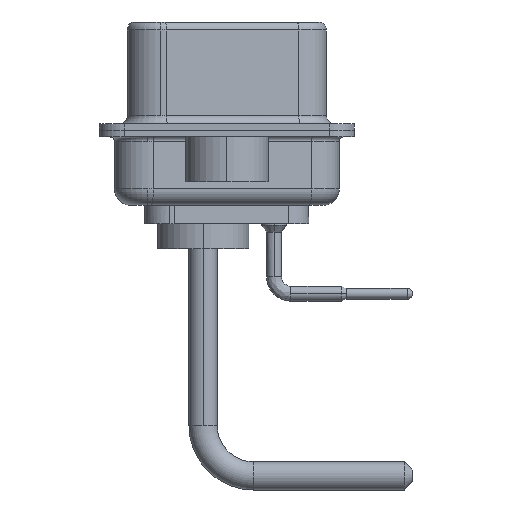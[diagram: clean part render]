
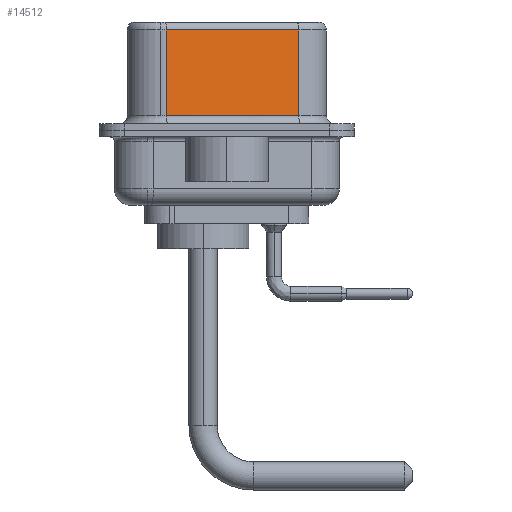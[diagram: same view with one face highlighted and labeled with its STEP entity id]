
A CAD part, left-side view. The second image highlights one B-rep face of the part: STEP entity #14512.
In plain terms, the highlighted planar face has unit normal (-0.985, -0.174, 0).
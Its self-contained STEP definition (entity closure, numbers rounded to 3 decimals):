
#419 = VERTEX_POINT ( 'NONE', #1103 ) ;
#1103 = CARTESIAN_POINT ( 'NONE',  ( 5.132, -4.322, 6.02 ) ) ;
#1244 = FACE_OUTER_BOUND ( 'NONE', #10131, .T. ) ;
#2244 = VERTEX_POINT ( 'NONE', #3021 ) ;
#2756 = VERTEX_POINT ( 'NONE', #20023 ) ;
#3021 = CARTESIAN_POINT ( 'NONE',  ( 3.73, 3.628, 6.02 ) ) ;
#3623 = ORIENTED_EDGE ( 'NONE', *, *, #19586, .T. ) ;
#5337 = ORIENTED_EDGE ( 'NONE', *, *, #9830, .T. ) ;
#7617 = LINE ( 'NONE', #9906, #19310 ) ;
#7746 = DIRECTION ( 'NONE',  ( 0.174, -0.985, 0. ) ) ;
#8601 = CARTESIAN_POINT ( 'NONE',  ( 5.132, -4.322, 6.52 ) ) ;
#8750 = LINE ( 'NONE', #16131, #20574 ) ;
#9830 = EDGE_CURVE ( 'NONE', #419, #2244, #7617, .T. ) ;
#9906 = CARTESIAN_POINT ( 'NONE',  ( 5.132, -4.322, 6.02 ) ) ;
#10066 = PLANE ( 'NONE',  #12535 ) ;
#10131 = EDGE_LOOP ( 'NONE', ( #11204, #5337, #3623, #23780 ) ) ;
#11204 = ORIENTED_EDGE ( 'NONE', *, *, #15898, .F. ) ;
#11351 = CARTESIAN_POINT ( 'NONE',  ( 5.132, -4.322, 6.52 ) ) ;
#12423 = EDGE_CURVE ( 'NONE', #2756, #22109, #8750, .T. ) ;
#12535 = AXIS2_PLACEMENT_3D ( 'NONE', #8601, #23154, #23276 ) ;
#14103 = VECTOR ( 'NONE', #15091, 1000. ) ;
#14512 = ADVANCED_FACE ( 'NONE', ( #1244 ), #10066, .F. ) ;
#15091 = DIRECTION ( 'NONE',  ( 0., 0., -1. ) ) ;
#15898 = EDGE_CURVE ( 'NONE', #419, #22109, #18730, .T. ) ;
#16131 = CARTESIAN_POINT ( 'NONE',  ( 5.132, -4.322, 0.9 ) ) ;
#16332 = DIRECTION ( 'NONE',  ( 0., 0., -1. ) ) ;
#18328 = CARTESIAN_POINT ( 'NONE',  ( 5.132, -4.322, 0.9 ) ) ;
#18730 = LINE ( 'NONE', #11351, #14103 ) ;
#18744 = DIRECTION ( 'NONE',  ( -0.174, 0.985, 0. ) ) ;
#19310 = VECTOR ( 'NONE', #18744, 1000. ) ;
#19586 = EDGE_CURVE ( 'NONE', #2244, #2756, #22791, .T. ) ;
#19628 = VECTOR ( 'NONE', #16332, 1000. ) ;
#20023 = CARTESIAN_POINT ( 'NONE',  ( 3.73, 3.628, 0.9 ) ) ;
#20574 = VECTOR ( 'NONE', #7746, 1000. ) ;
#22109 = VERTEX_POINT ( 'NONE', #18328 ) ;
#22791 = LINE ( 'NONE', #22919, #19628 ) ;
#22919 = CARTESIAN_POINT ( 'NONE',  ( 3.73, 3.628, 6.52 ) ) ;
#23154 = DIRECTION ( 'NONE',  ( 0.985, 0.174, 0. ) ) ;
#23276 = DIRECTION ( 'NONE',  ( -0.174, 0.985, 0. ) ) ;
#23780 = ORIENTED_EDGE ( 'NONE', *, *, #12423, .T. ) ;
